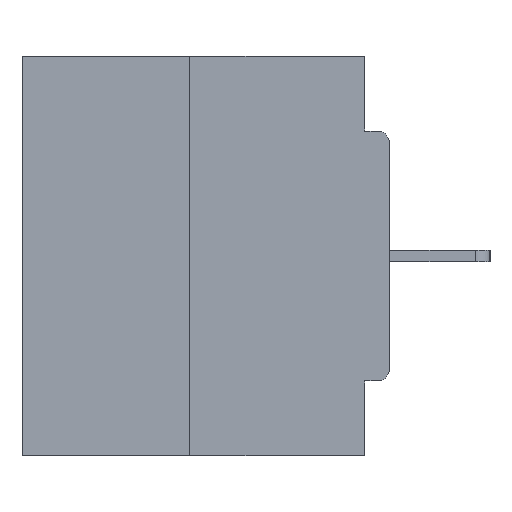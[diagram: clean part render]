
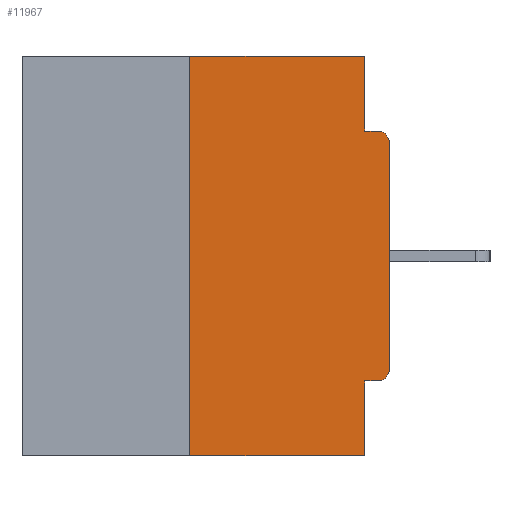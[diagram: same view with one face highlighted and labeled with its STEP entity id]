
A CAD part, left-side view. The second image highlights one B-rep face of the part: STEP entity #11967.
In plain terms, the highlighted planar face has unit normal (-1, 0, 0).
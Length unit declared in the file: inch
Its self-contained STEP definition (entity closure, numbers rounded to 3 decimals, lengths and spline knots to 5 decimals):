
#18 = ORIENTED_EDGE ( 'NONE', *, *, #21100, .F. ) ;
#97 = VECTOR ( 'NONE', #21251, 39.37008 ) ;
#554 = VERTEX_POINT ( 'NONE', #30903 ) ;
#791 = EDGE_CURVE ( 'NONE', #8896, #13310, #11769, .T. ) ;
#1033 = VECTOR ( 'NONE', #22848, 39.37008 ) ;
#1544 = VECTOR ( 'NONE', #8805, 39.37008 ) ;
#2603 = CARTESIAN_POINT ( 'NONE',  ( 0., 0.25, -0.5 ) ) ;
#3779 = LINE ( 'NONE', #15112, #20424 ) ;
#4085 = DIRECTION ( 'NONE',  ( -1., 0., 0. ) ) ;
#4295 = DIRECTION ( 'NONE',  ( 0., 0., -1. ) ) ;
#4340 = ORIENTED_EDGE ( 'NONE', *, *, #16537, .F. ) ;
#5258 = AXIS2_PLACEMENT_3D ( 'NONE', #18859, #21217, #28493 ) ;
#5696 = ORIENTED_EDGE ( 'NONE', *, *, #22479, .F. ) ;
#5973 = EDGE_CURVE ( 'NONE', #13310, #20099, #7390, .T. ) ;
#6323 = EDGE_CURVE ( 'NONE', #20630, #21018, #12811, .T. ) ;
#6466 = EDGE_CURVE ( 'NONE', #14132, #20099, #10756, .T. ) ;
#7150 = FACE_OUTER_BOUND ( 'NONE', #7450, .T. ) ;
#7390 = LINE ( 'NONE', #16687, #97 ) ;
#7450 = EDGE_LOOP ( 'NONE', ( #4340, #22331, #19355, #5696, #18, #21630, #22322, #22829, #27921, #22568 ) ) ;
#8805 = DIRECTION ( 'NONE',  ( 0., 1., 0. ) ) ;
#8896 = VERTEX_POINT ( 'NONE', #18169 ) ;
#9000 = CARTESIAN_POINT ( 'NONE',  ( 0., 0.031, -0.5 ) ) ;
#9092 = CARTESIAN_POINT ( 'NONE',  ( 0., 0.031, 0. ) ) ;
#9261 = DIRECTION ( 'NONE',  ( 0., 0., 1. ) ) ;
#10756 = CIRCLE ( 'NONE', #5258, 0.015 ) ;
#11295 = DIRECTION ( 'NONE',  ( 0., 0., -1. ) ) ;
#11769 = LINE ( 'NONE', #9092, #1033 ) ;
#11967 = ADVANCED_FACE ( 'NONE', ( #7150 ), #29342, .F. ) ;
#12487 = DIRECTION ( 'NONE',  ( 0., 0., -1. ) ) ;
#12508 = CARTESIAN_POINT ( 'NONE',  ( 0., 0.46, 0. ) ) ;
#12811 = CIRCLE ( 'NONE', #17855, 0.015 ) ;
#13310 = VERTEX_POINT ( 'NONE', #26677 ) ;
#14132 = VERTEX_POINT ( 'NONE', #19195 ) ;
#14436 = VERTEX_POINT ( 'NONE', #18543 ) ;
#15080 = CARTESIAN_POINT ( 'NONE',  ( 0., 0.015, -0.0935 ) ) ;
#15112 = CARTESIAN_POINT ( 'NONE',  ( 0., 0.46, -0.5 ) ) ;
#15266 = DIRECTION ( 'NONE',  ( 0., -1., 0. ) ) ;
#15741 = EDGE_CURVE ( 'NONE', #16841, #14436, #3779, .T. ) ;
#15899 = LINE ( 'NONE', #30074, #1544 ) ;
#16040 = CARTESIAN_POINT ( 'NONE',  ( 0., 0.015, -0.3915 ) ) ;
#16098 = LINE ( 'NONE', #9000, #19168 ) ;
#16159 = CARTESIAN_POINT ( 'NONE',  ( 0., 0.25, 0. ) ) ;
#16362 = CARTESIAN_POINT ( 'NONE',  ( 0., 0., 0. ) ) ;
#16537 = EDGE_CURVE ( 'NONE', #23162, #8896, #29684, .T. ) ;
#16687 = CARTESIAN_POINT ( 'NONE',  ( 0., 0., -0.0935 ) ) ;
#16841 = VERTEX_POINT ( 'NONE', #2603 ) ;
#17064 = DIRECTION ( 'NONE',  ( 1., 0., 0. ) ) ;
#17388 = DIRECTION ( 'NONE',  ( 0., -1., 0. ) ) ;
#17855 = AXIS2_PLACEMENT_3D ( 'NONE', #16040, #4085, #11295 ) ;
#18169 = CARTESIAN_POINT ( 'NONE',  ( 0., 0.031, 0. ) ) ;
#18403 = LINE ( 'NONE', #16362, #21407 ) ;
#18543 = CARTESIAN_POINT ( 'NONE',  ( 0., 0.031, -0.5 ) ) ;
#18859 = CARTESIAN_POINT ( 'NONE',  ( 0., 0.015, -0.1085 ) ) ;
#18872 = VECTOR ( 'NONE', #27633, 39.37008 ) ;
#19168 = VECTOR ( 'NONE', #4295, 39.37008 ) ;
#19195 = CARTESIAN_POINT ( 'NONE',  ( 0., 0., -0.1085 ) ) ;
#19355 = ORIENTED_EDGE ( 'NONE', *, *, #15741, .T. ) ;
#20099 = VERTEX_POINT ( 'NONE', #15080 ) ;
#20217 = AXIS2_PLACEMENT_3D ( 'NONE', #22241, #17064, #12487 ) ;
#20424 = VECTOR ( 'NONE', #15266, 39.37008 ) ;
#20630 = VERTEX_POINT ( 'NONE', #22270 ) ;
#20845 = CARTESIAN_POINT ( 'NONE',  ( 0., 0.25, 0. ) ) ;
#21018 = VERTEX_POINT ( 'NONE', #27880 ) ;
#21100 = EDGE_CURVE ( 'NONE', #20630, #554, #15899, .T. ) ;
#21217 = DIRECTION ( 'NONE',  ( -1., 0., 0. ) ) ;
#21251 = DIRECTION ( 'NONE',  ( 0., -1., 0. ) ) ;
#21407 = VECTOR ( 'NONE', #9261, 39.37008 ) ;
#21630 = ORIENTED_EDGE ( 'NONE', *, *, #6323, .T. ) ;
#22241 = CARTESIAN_POINT ( 'NONE',  ( 0., 0.46, 0. ) ) ;
#22270 = CARTESIAN_POINT ( 'NONE',  ( 0., 0.015, -0.4065 ) ) ;
#22322 = ORIENTED_EDGE ( 'NONE', *, *, #29376, .T. ) ;
#22331 = ORIENTED_EDGE ( 'NONE', *, *, #28848, .F. ) ;
#22479 = EDGE_CURVE ( 'NONE', #554, #14436, #16098, .T. ) ;
#22568 = ORIENTED_EDGE ( 'NONE', *, *, #791, .F. ) ;
#22829 = ORIENTED_EDGE ( 'NONE', *, *, #6466, .T. ) ;
#22848 = DIRECTION ( 'NONE',  ( 0., 0., -1. ) ) ;
#23162 = VERTEX_POINT ( 'NONE', #16159 ) ;
#26493 = VECTOR ( 'NONE', #17388, 39.37008 ) ;
#26677 = CARTESIAN_POINT ( 'NONE',  ( 0., 0.031, -0.0935 ) ) ;
#27633 = DIRECTION ( 'NONE',  ( 0., 0., 1. ) ) ;
#27880 = CARTESIAN_POINT ( 'NONE',  ( 0., 0., -0.3915 ) ) ;
#27921 = ORIENTED_EDGE ( 'NONE', *, *, #5973, .F. ) ;
#28493 = DIRECTION ( 'NONE',  ( 0., 0., -1. ) ) ;
#28848 = EDGE_CURVE ( 'NONE', #16841, #23162, #30141, .T. ) ;
#29342 = PLANE ( 'NONE',  #20217 ) ;
#29376 = EDGE_CURVE ( 'NONE', #21018, #14132, #18403, .T. ) ;
#29684 = LINE ( 'NONE', #12508, #26493 ) ;
#30074 = CARTESIAN_POINT ( 'NONE',  ( 0., 0., -0.4065 ) ) ;
#30141 = LINE ( 'NONE', #20845, #18872 ) ;
#30903 = CARTESIAN_POINT ( 'NONE',  ( 0., 0.031, -0.4065 ) ) ;
